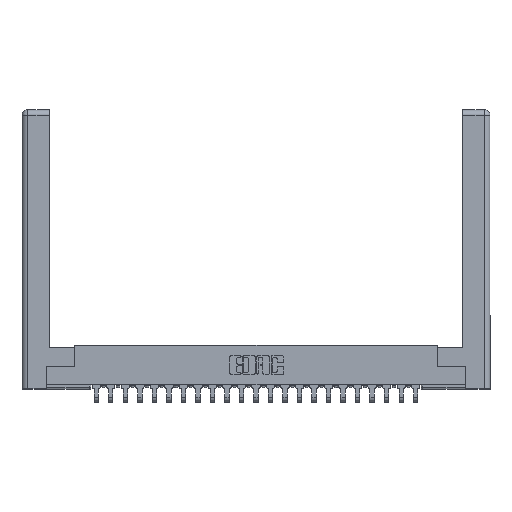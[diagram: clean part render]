
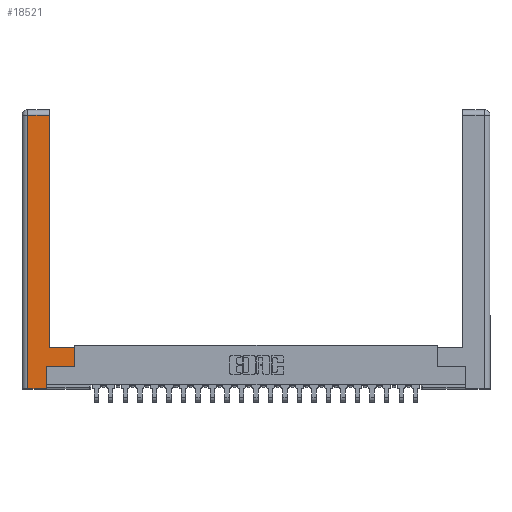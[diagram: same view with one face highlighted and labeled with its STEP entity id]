
A CAD part, top view. The second image highlights one B-rep face of the part: STEP entity #18521.
In plain terms, the highlighted planar face has unit normal (0, 0, 1).
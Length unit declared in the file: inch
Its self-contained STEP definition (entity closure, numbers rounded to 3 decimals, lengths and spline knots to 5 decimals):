
#274 = LINE ( 'NONE', #12230, #5953 ) ;
#339 = CARTESIAN_POINT ( 'NONE',  ( 0.265, 0.245, 0. ) ) ;
#1431 = ORIENTED_EDGE ( 'NONE', *, *, #3318, .T. ) ;
#1766 = ORIENTED_EDGE ( 'NONE', *, *, #14958, .T. ) ;
#2586 = CARTESIAN_POINT ( 'NONE',  ( 0.0615, 0., 0. ) ) ;
#3318 = EDGE_CURVE ( 'NONE', #20733, #15380, #8152, .T. ) ;
#3448 = ORIENTED_EDGE ( 'NONE', *, *, #12186, .T. ) ;
#3954 = EDGE_CURVE ( 'NONE', #8111, #5549, #10187, .T. ) ;
#3987 = CARTESIAN_POINT ( 'NONE',  ( 0.0615, 2.94, 0. ) ) ;
#4215 = VECTOR ( 'NONE', #9959, 39.37008 ) ;
#4405 = DIRECTION ( 'NONE',  ( -1., 0., 0. ) ) ;
#4607 = DIRECTION ( 'NONE',  ( -1., 0., 0. ) ) ;
#5221 = LINE ( 'NONE', #10101, #20210 ) ;
#5549 = VERTEX_POINT ( 'NONE', #16724 ) ;
#5776 = LINE ( 'NONE', #20982, #24030 ) ;
#5953 = VECTOR ( 'NONE', #19648, 39.37008 ) ;
#6153 = CARTESIAN_POINT ( 'NONE',  ( 0.565, 0.45, 0. ) ) ;
#6284 = PLANE ( 'NONE',  #8118 ) ;
#6350 = VECTOR ( 'NONE', #6556, 39.37008 ) ;
#6475 = CARTESIAN_POINT ( 'NONE',  ( 0.0615, 0., 0. ) ) ;
#6556 = DIRECTION ( 'NONE',  ( -1., 0., 0. ) ) ;
#8028 = LINE ( 'NONE', #9878, #13129 ) ;
#8111 = VERTEX_POINT ( 'NONE', #339 ) ;
#8118 = AXIS2_PLACEMENT_3D ( 'NONE', #19879, #14137, #4607 ) ;
#8152 = LINE ( 'NONE', #9758, #6350 ) ;
#9689 = ORIENTED_EDGE ( 'NONE', *, *, #10918, .T. ) ;
#9758 = CARTESIAN_POINT ( 'NONE',  ( 0.295, 0.45, 0. ) ) ;
#9878 = CARTESIAN_POINT ( 'NONE',  ( 0.565, 0.45, 0. ) ) ;
#9959 = DIRECTION ( 'NONE',  ( 1., 0., 0. ) ) ;
#10101 = CARTESIAN_POINT ( 'NONE',  ( 0.0615, 2.94, 0. ) ) ;
#10187 = LINE ( 'NONE', #19066, #4215 ) ;
#10534 = ORIENTED_EDGE ( 'NONE', *, *, #3954, .T. ) ;
#10918 = EDGE_CURVE ( 'NONE', #13540, #11976, #23381, .T. ) ;
#11381 = VERTEX_POINT ( 'NONE', #15955 ) ;
#11511 = DIRECTION ( 'NONE',  ( 0., 1., 0. ) ) ;
#11605 = CARTESIAN_POINT ( 'NONE',  ( 0.295, 0.45, 0. ) ) ;
#11661 = DIRECTION ( 'NONE',  ( 0., 1., 0. ) ) ;
#11976 = VERTEX_POINT ( 'NONE', #16968 ) ;
#12186 = EDGE_CURVE ( 'NONE', #15380, #11381, #274, .T. ) ;
#12230 = CARTESIAN_POINT ( 'NONE',  ( 0.295, 3., 0. ) ) ;
#12294 = DIRECTION ( 'NONE',  ( 1., 0., 0. ) ) ;
#13129 = VECTOR ( 'NONE', #11661, 39.37008 ) ;
#13540 = VERTEX_POINT ( 'NONE', #6475 ) ;
#14137 = DIRECTION ( 'NONE',  ( 0., 0., -1. ) ) ;
#14290 = CARTESIAN_POINT ( 'NONE',  ( 0.265, 0., 0. ) ) ;
#14892 = EDGE_CURVE ( 'NONE', #11381, #20663, #5221, .T. ) ;
#14958 = EDGE_CURVE ( 'NONE', #20663, #13540, #23802, .T. ) ;
#15326 = ORIENTED_EDGE ( 'NONE', *, *, #23784, .T. ) ;
#15380 = VERTEX_POINT ( 'NONE', #11605 ) ;
#15955 = CARTESIAN_POINT ( 'NONE',  ( 0.295, 2.94, 0. ) ) ;
#16724 = CARTESIAN_POINT ( 'NONE',  ( 0.565, 0.245, 0. ) ) ;
#16919 = VECTOR ( 'NONE', #21914, 39.37008 ) ;
#16968 = CARTESIAN_POINT ( 'NONE',  ( 0.265, 0., 0. ) ) ;
#18228 = EDGE_CURVE ( 'NONE', #11976, #8111, #5776, .T. ) ;
#18521 = ADVANCED_FACE ( 'NONE', ( #21341 ), #6284, .F. ) ;
#19042 = ORIENTED_EDGE ( 'NONE', *, *, #14892, .T. ) ;
#19066 = CARTESIAN_POINT ( 'NONE',  ( 0.565, 0.245, 0. ) ) ;
#19648 = DIRECTION ( 'NONE',  ( 0., 1., 0. ) ) ;
#19879 = CARTESIAN_POINT ( 'NONE',  ( 0., 0., 0. ) ) ;
#20210 = VECTOR ( 'NONE', #4405, 39.37008 ) ;
#20663 = VERTEX_POINT ( 'NONE', #3987 ) ;
#20733 = VERTEX_POINT ( 'NONE', #6153 ) ;
#20982 = CARTESIAN_POINT ( 'NONE',  ( 0.265, 0.245, 0. ) ) ;
#21323 = VECTOR ( 'NONE', #12294, 39.37008 ) ;
#21341 = FACE_OUTER_BOUND ( 'NONE', #24730, .T. ) ;
#21914 = DIRECTION ( 'NONE',  ( 0., -1., 0. ) ) ;
#22003 = ORIENTED_EDGE ( 'NONE', *, *, #18228, .T. ) ;
#23381 = LINE ( 'NONE', #14290, #21323 ) ;
#23784 = EDGE_CURVE ( 'NONE', #5549, #20733, #8028, .T. ) ;
#23802 = LINE ( 'NONE', #2586, #16919 ) ;
#24030 = VECTOR ( 'NONE', #11511, 39.37008 ) ;
#24730 = EDGE_LOOP ( 'NONE', ( #3448, #19042, #1766, #9689, #22003, #10534, #15326, #1431 ) ) ;
